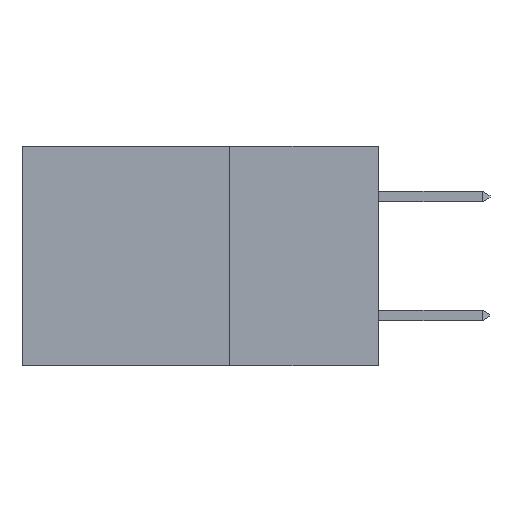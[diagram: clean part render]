
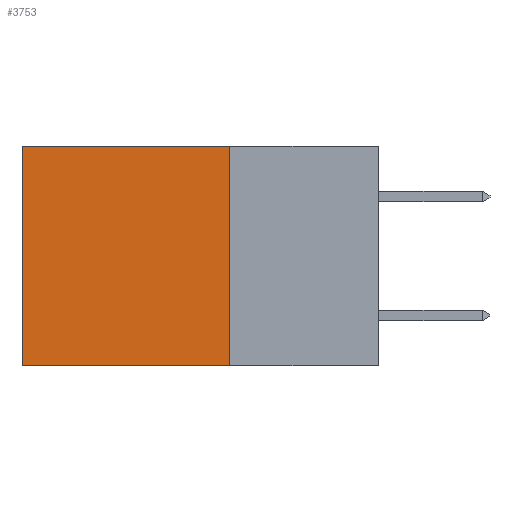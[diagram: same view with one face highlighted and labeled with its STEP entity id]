
A CAD part, left-side view. The second image highlights one B-rep face of the part: STEP entity #3753.
In plain terms, the highlighted planar face has unit normal (-1, 0, 0).
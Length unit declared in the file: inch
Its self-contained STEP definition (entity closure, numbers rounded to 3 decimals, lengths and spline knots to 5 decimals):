
#566 = FACE_OUTER_BOUND ( 'NONE', #3007, .T. ) ;
#1073 = LINE ( 'NONE', #8496, #8965 ) ;
#1108 = VECTOR ( 'NONE', #3962, 39.37008 ) ;
#1428 = CARTESIAN_POINT ( 'NONE',  ( 0.298, 0.25, -0.37 ) ) ;
#3007 = EDGE_LOOP ( 'NONE', ( #10622, #7255, #8073, #7139 ) ) ;
#3477 = LINE ( 'NONE', #8234, #11260 ) ;
#3490 = DIRECTION ( 'NONE',  ( 0., 1., 0. ) ) ;
#3508 = VERTEX_POINT ( 'NONE', #6689 ) ;
#3753 = ADVANCED_FACE ( 'NONE', ( #566 ), #12107, .F. ) ;
#3962 = DIRECTION ( 'NONE',  ( 0., 0., -1. ) ) ;
#5314 = VERTEX_POINT ( 'NONE', #12782 ) ;
#5465 = VERTEX_POINT ( 'NONE', #9027 ) ;
#6599 = LINE ( 'NONE', #13069, #1108 ) ;
#6689 = CARTESIAN_POINT ( 'NONE',  ( 0.298, 0.6, -0.37 ) ) ;
#6778 = EDGE_CURVE ( 'NONE', #5465, #5314, #6599, .T. ) ;
#7139 = ORIENTED_EDGE ( 'NONE', *, *, #10246, .T. ) ;
#7255 = ORIENTED_EDGE ( 'NONE', *, *, #9750, .F. ) ;
#7620 = AXIS2_PLACEMENT_3D ( 'NONE', #12117, #12161, #12159 ) ;
#8073 = ORIENTED_EDGE ( 'NONE', *, *, #6778, .F. ) ;
#8234 = CARTESIAN_POINT ( 'NONE',  ( 0.298, 0.6, 0. ) ) ;
#8496 = CARTESIAN_POINT ( 'NONE',  ( 0.298, 0.25, 0. ) ) ;
#8819 = EDGE_CURVE ( 'NONE', #11687, #3508, #3477, .T. ) ;
#8965 = VECTOR ( 'NONE', #12454, 39.37008 ) ;
#9027 = CARTESIAN_POINT ( 'NONE',  ( 0.298, 0.25, 0. ) ) ;
#9200 = DIRECTION ( 'NONE',  ( 0., 0., -1. ) ) ;
#9750 = EDGE_CURVE ( 'NONE', #5314, #3508, #9985, .T. ) ;
#9985 = LINE ( 'NONE', #1428, #12708 ) ;
#10246 = EDGE_CURVE ( 'NONE', #5465, #11687, #1073, .T. ) ;
#10622 = ORIENTED_EDGE ( 'NONE', *, *, #8819, .T. ) ;
#11260 = VECTOR ( 'NONE', #9200, 39.37008 ) ;
#11687 = VERTEX_POINT ( 'NONE', #13211 ) ;
#12107 = PLANE ( 'NONE',  #7620 ) ;
#12117 = CARTESIAN_POINT ( 'NONE',  ( 0.298, 0.25, 0. ) ) ;
#12159 = DIRECTION ( 'NONE',  ( 0., 0., -1. ) ) ;
#12161 = DIRECTION ( 'NONE',  ( 1., 0., 0. ) ) ;
#12454 = DIRECTION ( 'NONE',  ( 0., 1., 0. ) ) ;
#12708 = VECTOR ( 'NONE', #3490, 39.37008 ) ;
#12782 = CARTESIAN_POINT ( 'NONE',  ( 0.298, 0.25, -0.37 ) ) ;
#13069 = CARTESIAN_POINT ( 'NONE',  ( 0.298, 0.25, 0. ) ) ;
#13211 = CARTESIAN_POINT ( 'NONE',  ( 0.298, 0.6, 0. ) ) ;
